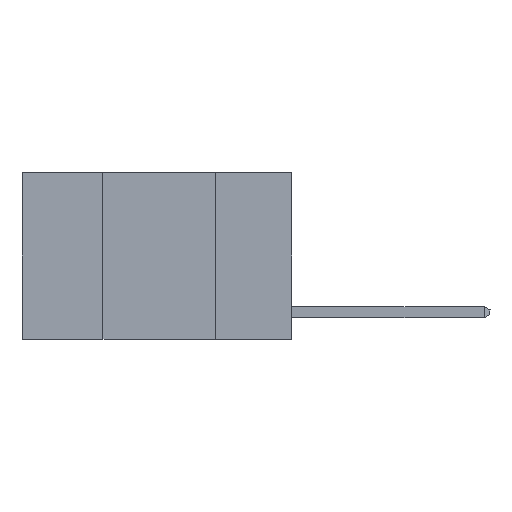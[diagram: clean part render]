
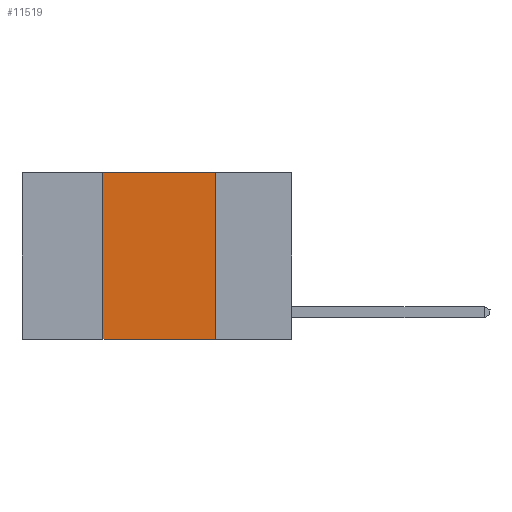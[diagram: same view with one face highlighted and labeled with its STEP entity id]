
A CAD part, left-side view. The second image highlights one B-rep face of the part: STEP entity #11519.
In plain terms, the highlighted planar face has unit normal (-1, 0, 0).
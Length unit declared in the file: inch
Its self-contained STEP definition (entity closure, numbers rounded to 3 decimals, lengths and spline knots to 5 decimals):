
#368 = DIRECTION ( 'NONE',  ( 0., -1., 0. ) ) ;
#525 = VECTOR ( 'NONE', #368, 39.37008 ) ;
#694 = VERTEX_POINT ( 'NONE', #3705 ) ;
#1129 = DIRECTION ( 'NONE',  ( 0., 0., 1. ) ) ;
#1858 = ORIENTED_EDGE ( 'NONE', *, *, #15986, .T. ) ;
#2209 = DIRECTION ( 'NONE',  ( 1., 0., 0. ) ) ;
#3705 = CARTESIAN_POINT ( 'NONE',  ( 0., 0.42, 0. ) ) ;
#4242 = LINE ( 'NONE', #11371, #525 ) ;
#5138 = VECTOR ( 'NONE', #13005, 39.37008 ) ;
#5751 = DIRECTION ( 'NONE',  ( 0., -1., 0. ) ) ;
#5816 = ORIENTED_EDGE ( 'NONE', *, *, #9386, .F. ) ;
#6127 = VECTOR ( 'NONE', #5751, 39.37008 ) ;
#6235 = ORIENTED_EDGE ( 'NONE', *, *, #14600, .F. ) ;
#6392 = PLANE ( 'NONE',  #17287 ) ;
#6524 = VERTEX_POINT ( 'NONE', #13656 ) ;
#7149 = CARTESIAN_POINT ( 'NONE',  ( 0., 0.6, -0.37 ) ) ;
#7271 = VERTEX_POINT ( 'NONE', #15092 ) ;
#7685 = EDGE_CURVE ( 'NONE', #6524, #694, #8969, .T. ) ;
#8969 = LINE ( 'NONE', #10748, #9819 ) ;
#9386 = EDGE_CURVE ( 'NONE', #7271, #12535, #15769, .T. ) ;
#9754 = LINE ( 'NONE', #7149, #6127 ) ;
#9819 = VECTOR ( 'NONE', #1129, 39.37008 ) ;
#10465 = CARTESIAN_POINT ( 'NONE',  ( 0., 0.6, 0. ) ) ;
#10748 = CARTESIAN_POINT ( 'NONE',  ( 0., 0.42, 0. ) ) ;
#11371 = CARTESIAN_POINT ( 'NONE',  ( 0., 0.6, 0. ) ) ;
#11519 = ADVANCED_FACE ( 'NONE', ( #15071 ), #6392, .F. ) ;
#11775 = DIRECTION ( 'NONE',  ( 0., 0., -1. ) ) ;
#12363 = CARTESIAN_POINT ( 'NONE',  ( 0., 0.17, -0.37 ) ) ;
#12535 = VERTEX_POINT ( 'NONE', #12363 ) ;
#13005 = DIRECTION ( 'NONE',  ( 0., 0., -1. ) ) ;
#13656 = CARTESIAN_POINT ( 'NONE',  ( 0., 0.42, -0.37 ) ) ;
#14600 = EDGE_CURVE ( 'NONE', #694, #7271, #4242, .T. ) ;
#15071 = FACE_OUTER_BOUND ( 'NONE', #16947, .T. ) ;
#15092 = CARTESIAN_POINT ( 'NONE',  ( 0., 0.17, 0. ) ) ;
#15380 = ORIENTED_EDGE ( 'NONE', *, *, #7685, .F. ) ;
#15769 = LINE ( 'NONE', #16868, #5138 ) ;
#15986 = EDGE_CURVE ( 'NONE', #6524, #12535, #9754, .T. ) ;
#16868 = CARTESIAN_POINT ( 'NONE',  ( 0., 0.17, 0. ) ) ;
#16947 = EDGE_LOOP ( 'NONE', ( #5816, #6235, #15380, #1858 ) ) ;
#17287 = AXIS2_PLACEMENT_3D ( 'NONE', #10465, #2209, #11775 ) ;
